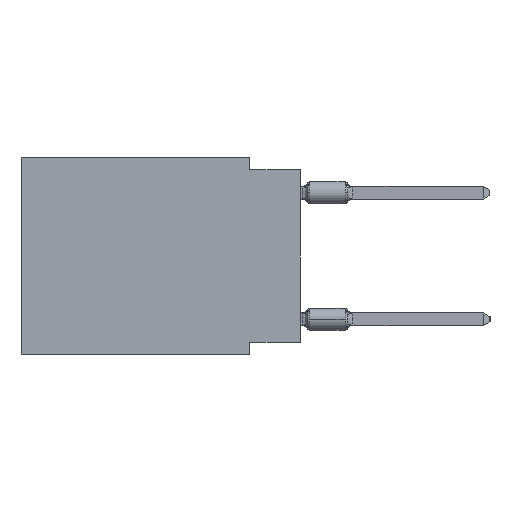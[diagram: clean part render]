
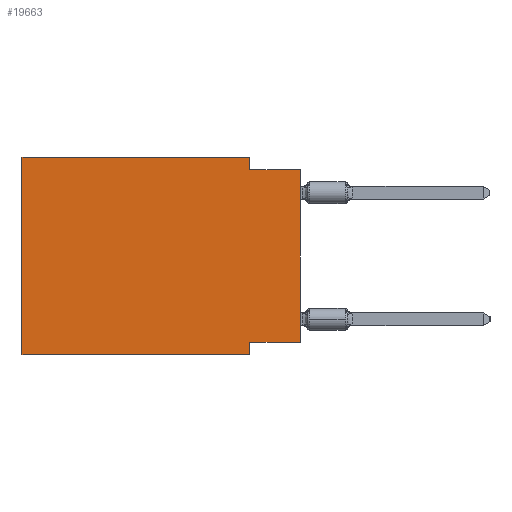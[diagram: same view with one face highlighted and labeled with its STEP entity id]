
A CAD part, left-side view. The second image highlights one B-rep face of the part: STEP entity #19663.
In plain terms, the highlighted planar face has unit normal (-1, 0, 0).
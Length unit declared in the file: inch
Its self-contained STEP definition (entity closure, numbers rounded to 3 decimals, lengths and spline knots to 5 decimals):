
#837 = EDGE_CURVE ( 'NONE', #13416, #4467, #19594, .T. ) ;
#1002 = DIRECTION ( 'NONE',  ( 1., 0., 0. ) ) ;
#1495 = DIRECTION ( 'NONE',  ( 0., 0., -1. ) ) ;
#2161 = EDGE_CURVE ( 'NONE', #20468, #23230, #23116, .T. ) ;
#2243 = ORIENTED_EDGE ( 'NONE', *, *, #31860, .F. ) ;
#4467 = VERTEX_POINT ( 'NONE', #21567 ) ;
#5192 = CARTESIAN_POINT ( 'NONE',  ( 0., 0., -0.025 ) ) ;
#5714 = DIRECTION ( 'NONE',  ( 0., 0., -1. ) ) ;
#5784 = VERTEX_POINT ( 'NONE', #21255 ) ;
#6250 = FACE_OUTER_BOUND ( 'NONE', #31656, .T. ) ;
#7961 = DIRECTION ( 'NONE',  ( 0., -1., 0. ) ) ;
#9623 = VECTOR ( 'NONE', #7961, 39.37008 ) ;
#9701 = ORIENTED_EDGE ( 'NONE', *, *, #19901, .T. ) ;
#10446 = VERTEX_POINT ( 'NONE', #5192 ) ;
#10694 = VECTOR ( 'NONE', #29749, 39.37008 ) ;
#10764 = EDGE_CURVE ( 'NONE', #4467, #20468, #25251, .T. ) ;
#10964 = CARTESIAN_POINT ( 'NONE',  ( 0., 0., 0. ) ) ;
#11346 = DIRECTION ( 'NONE',  ( 0., 0., 1. ) ) ;
#13007 = CARTESIAN_POINT ( 'NONE',  ( 0., 0.55, -0.39 ) ) ;
#13416 = VERTEX_POINT ( 'NONE', #13007 ) ;
#13472 = DIRECTION ( 'NONE',  ( 0., -1., 0. ) ) ;
#14534 = AXIS2_PLACEMENT_3D ( 'NONE', #27493, #1002, #30194 ) ;
#14709 = CARTESIAN_POINT ( 'NONE',  ( 0., 0.55, -0.39 ) ) ;
#16182 = VECTOR ( 'NONE', #19776, 39.37008 ) ;
#16208 = LINE ( 'NONE', #30678, #33462 ) ;
#16435 = VECTOR ( 'NONE', #11346, 39.37008 ) ;
#18221 = CARTESIAN_POINT ( 'NONE',  ( 0., 0., -0.365 ) ) ;
#19594 = LINE ( 'NONE', #37337, #16182 ) ;
#19663 = ADVANCED_FACE ( 'NONE', ( #6250 ), #21705, .F. ) ;
#19776 = DIRECTION ( 'NONE',  ( 0., 0., 1. ) ) ;
#19901 = EDGE_CURVE ( 'NONE', #13416, #5784, #31722, .T. ) ;
#19926 = CARTESIAN_POINT ( 'NONE',  ( 0., 0.1, -0.025 ) ) ;
#20468 = VERTEX_POINT ( 'NONE', #33192 ) ;
#20810 = EDGE_CURVE ( 'NONE', #26892, #10446, #26028, .T. ) ;
#20919 = CARTESIAN_POINT ( 'NONE',  ( 0., 0., -0.025 ) ) ;
#21255 = CARTESIAN_POINT ( 'NONE',  ( 0., 0.1, -0.39 ) ) ;
#21567 = CARTESIAN_POINT ( 'NONE',  ( 0., 0.55, 0. ) ) ;
#21705 = PLANE ( 'NONE',  #14534 ) ;
#22830 = CARTESIAN_POINT ( 'NONE',  ( 0., 0.1, -0.365 ) ) ;
#23116 = LINE ( 'NONE', #37578, #28899 ) ;
#23230 = VERTEX_POINT ( 'NONE', #19926 ) ;
#24142 = ORIENTED_EDGE ( 'NONE', *, *, #837, .F. ) ;
#24474 = VERTEX_POINT ( 'NONE', #22830 ) ;
#24707 = VECTOR ( 'NONE', #13472, 39.37008 ) ;
#25251 = LINE ( 'NONE', #33746, #24707 ) ;
#26028 = LINE ( 'NONE', #10964, #16435 ) ;
#26892 = VERTEX_POINT ( 'NONE', #18221 ) ;
#26900 = EDGE_CURVE ( 'NONE', #23230, #10446, #27096, .T. ) ;
#27096 = LINE ( 'NONE', #20919, #35788 ) ;
#27493 = CARTESIAN_POINT ( 'NONE',  ( 0., 0.55, 0. ) ) ;
#28399 = ORIENTED_EDGE ( 'NONE', *, *, #2161, .F. ) ;
#28899 = VECTOR ( 'NONE', #5714, 39.37008 ) ;
#29749 = DIRECTION ( 'NONE',  ( 0., 1., 0. ) ) ;
#30194 = DIRECTION ( 'NONE',  ( 0., 0., -1. ) ) ;
#30678 = CARTESIAN_POINT ( 'NONE',  ( 0., 0.1, -0.39 ) ) ;
#30940 = CARTESIAN_POINT ( 'NONE',  ( 0., 0., -0.365 ) ) ;
#31101 = ORIENTED_EDGE ( 'NONE', *, *, #34548, .F. ) ;
#31656 = EDGE_LOOP ( 'NONE', ( #33818, #32484, #28399, #31793, #24142, #9701, #2243, #31101 ) ) ;
#31722 = LINE ( 'NONE', #14709, #9623 ) ;
#31793 = ORIENTED_EDGE ( 'NONE', *, *, #10764, .F. ) ;
#31860 = EDGE_CURVE ( 'NONE', #24474, #5784, #16208, .T. ) ;
#32320 = DIRECTION ( 'NONE',  ( 0., -1., 0. ) ) ;
#32484 = ORIENTED_EDGE ( 'NONE', *, *, #26900, .F. ) ;
#33192 = CARTESIAN_POINT ( 'NONE',  ( 0., 0.1, 0. ) ) ;
#33462 = VECTOR ( 'NONE', #1495, 39.37008 ) ;
#33746 = CARTESIAN_POINT ( 'NONE',  ( 0., 0.55, 0. ) ) ;
#33818 = ORIENTED_EDGE ( 'NONE', *, *, #20810, .T. ) ;
#33823 = LINE ( 'NONE', #30940, #10694 ) ;
#34548 = EDGE_CURVE ( 'NONE', #26892, #24474, #33823, .T. ) ;
#35788 = VECTOR ( 'NONE', #32320, 39.37008 ) ;
#37337 = CARTESIAN_POINT ( 'NONE',  ( 0., 0.55, 0. ) ) ;
#37578 = CARTESIAN_POINT ( 'NONE',  ( 0., 0.1, 0. ) ) ;
